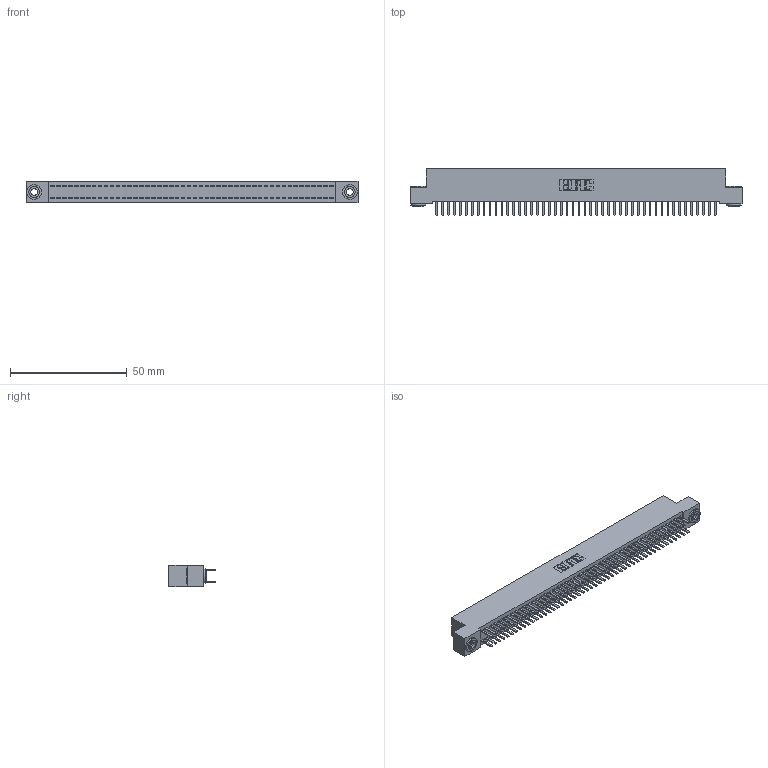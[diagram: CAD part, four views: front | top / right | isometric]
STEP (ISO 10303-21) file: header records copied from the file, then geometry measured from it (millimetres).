
FILE_DESCRIPTION (( 'STEP AP203' ), '1' );
FILE_NAME ('342-096-520-203.STEP', '2019-10-04T15:52:13', ( '' ), ( '' ), 'SwSTEP 2.0', 'SolidWorks 2016', '' );
FILE_SCHEMA (( 'CONFIG_CONTROL_DESIGN' ));
Length unit declared in the file: inch
Products named in the file (4): 345-292-001_345-293-120; 342-250-002_345-250-002-102; 342-096-520-203; 342 Part_.156 TH
Assembly tree (99 placements, depth 2):
  342-096-520-203
    342 Part_.156 TH
    345-292-001_345-293-120  x96
    342-250-002_345-250-002-102  x2
Bounding box: 142.24 x 20.02 x 9.4 mm (x, y, z)
Volume: 12789.3 mm3; surface area: 21080.1 mm2
Topology: 99 solids, 99 shells, 5524 faces, 16023 edges, 10422 vertices
Faces by surface type: plane 3724, cylinder 1792, cone 8
Entity records: 30736 total; most frequent: CARTESIAN_POINT 5073, ORIENTED_EDGE 4990, DIRECTION 4345, EDGE_CURVE 2495, VECTOR 2339, LINE 2339, VERTEX_POINT 1658, AXIS2_PLACEMENT_3D 1003
